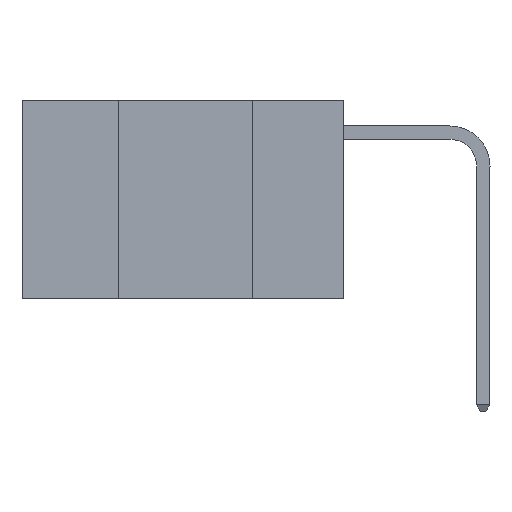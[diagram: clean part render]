
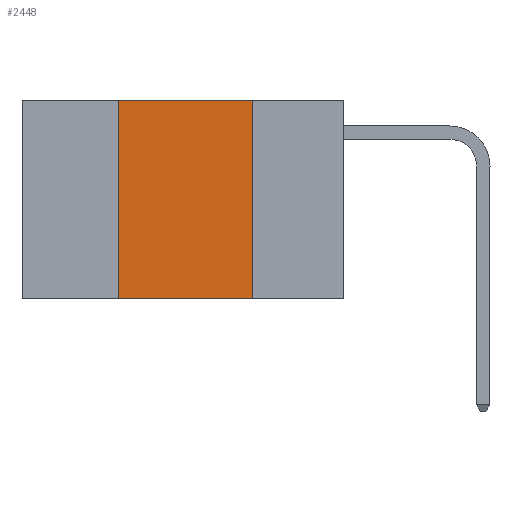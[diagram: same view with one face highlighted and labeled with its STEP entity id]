
A CAD part, left-side view. The second image highlights one B-rep face of the part: STEP entity #2448.
In plain terms, the highlighted planar face has unit normal (-1, 0, 0).
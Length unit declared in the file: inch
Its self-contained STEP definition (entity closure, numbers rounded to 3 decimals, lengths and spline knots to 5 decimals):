
#421 = VECTOR ( 'NONE', #6416, 39.37008 ) ;
#549 = PLANE ( 'NONE',  #9103 ) ;
#634 = CARTESIAN_POINT ( 'NONE',  ( 0., 0.17, 0. ) ) ;
#894 = CARTESIAN_POINT ( 'NONE',  ( 0., 0.42, 0. ) ) ;
#1183 = VECTOR ( 'NONE', #1386, 39.37008 ) ;
#1386 = DIRECTION ( 'NONE',  ( 0., -1., 0. ) ) ;
#1391 = DIRECTION ( 'NONE',  ( 0., 0., -1. ) ) ;
#1731 = DIRECTION ( 'NONE',  ( 0., 0., 1. ) ) ;
#2448 = ADVANCED_FACE ( 'NONE', ( #10294 ), #549, .F. ) ;
#2835 = ORIENTED_EDGE ( 'NONE', *, *, #9437, .F. ) ;
#2848 = VECTOR ( 'NONE', #4714, 39.37008 ) ;
#3119 = CARTESIAN_POINT ( 'NONE',  ( 0., 0.17, 0. ) ) ;
#3239 = CARTESIAN_POINT ( 'NONE',  ( 0., 0.42, -0.37 ) ) ;
#3706 = EDGE_CURVE ( 'NONE', #9677, #9454, #5022, .T. ) ;
#3792 = CARTESIAN_POINT ( 'NONE',  ( 0., 0.6, 0. ) ) ;
#4066 = EDGE_LOOP ( 'NONE', ( #2835, #6205, #7161, #5943 ) ) ;
#4568 = EDGE_CURVE ( 'NONE', #7216, #5555, #7667, .T. ) ;
#4658 = CARTESIAN_POINT ( 'NONE',  ( 0., 0.6, -0.37 ) ) ;
#4714 = DIRECTION ( 'NONE',  ( 0., 0., -1. ) ) ;
#4788 = CARTESIAN_POINT ( 'NONE',  ( 0., 0.6, 0. ) ) ;
#5022 = LINE ( 'NONE', #4788, #421 ) ;
#5271 = LINE ( 'NONE', #634, #2848 ) ;
#5555 = VERTEX_POINT ( 'NONE', #7527 ) ;
#5806 = VECTOR ( 'NONE', #1731, 39.37008 ) ;
#5943 = ORIENTED_EDGE ( 'NONE', *, *, #4568, .T. ) ;
#6205 = ORIENTED_EDGE ( 'NONE', *, *, #3706, .F. ) ;
#6254 = DIRECTION ( 'NONE',  ( 1., 0., 0. ) ) ;
#6416 = DIRECTION ( 'NONE',  ( 0., -1., 0. ) ) ;
#7161 = ORIENTED_EDGE ( 'NONE', *, *, #7827, .F. ) ;
#7216 = VERTEX_POINT ( 'NONE', #3239 ) ;
#7527 = CARTESIAN_POINT ( 'NONE',  ( 0., 0.17, -0.37 ) ) ;
#7667 = LINE ( 'NONE', #4658, #1183 ) ;
#7827 = EDGE_CURVE ( 'NONE', #7216, #9677, #10074, .T. ) ;
#8260 = CARTESIAN_POINT ( 'NONE',  ( 0., 0.42, 0. ) ) ;
#9103 = AXIS2_PLACEMENT_3D ( 'NONE', #3792, #6254, #1391 ) ;
#9437 = EDGE_CURVE ( 'NONE', #9454, #5555, #5271, .T. ) ;
#9454 = VERTEX_POINT ( 'NONE', #3119 ) ;
#9677 = VERTEX_POINT ( 'NONE', #8260 ) ;
#10074 = LINE ( 'NONE', #894, #5806 ) ;
#10294 = FACE_OUTER_BOUND ( 'NONE', #4066, .T. ) ;
